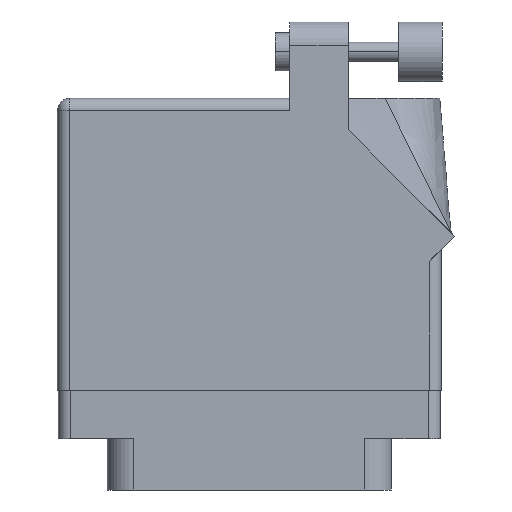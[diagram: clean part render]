
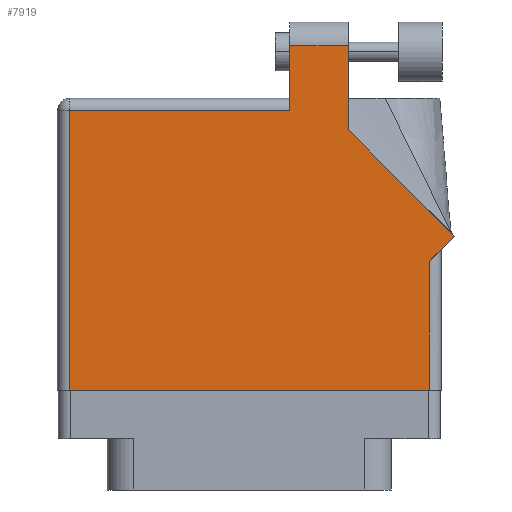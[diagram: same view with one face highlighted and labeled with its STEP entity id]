
A CAD part, front view. The second image highlights one B-rep face of the part: STEP entity #7919.
In plain terms, the highlighted face is planar.
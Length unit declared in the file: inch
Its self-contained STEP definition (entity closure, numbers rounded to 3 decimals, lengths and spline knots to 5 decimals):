
#289 = LINE ( 'NONE', #7121, #29170 ) ;
#647 = CARTESIAN_POINT ( 'NONE',  ( 0.943, 0.575, 0.455 ) ) ;
#1535 = CARTESIAN_POINT ( 'NONE',  ( -1.005, -0.1, 0.455 ) ) ;
#1773 = VECTOR ( 'NONE', #12366, 39.37008 ) ;
#2554 = ORIENTED_EDGE ( 'NONE', *, *, #29920, .T. ) ;
#2751 = CARTESIAN_POINT ( 'NONE',  ( 0.943, -0.1, 0.455 ) ) ;
#2792 = ORIENTED_EDGE ( 'NONE', *, *, #33206, .T. ) ;
#2858 = VECTOR ( 'NONE', #15403, 39.37008 ) ;
#3073 = CARTESIAN_POINT ( 'NONE',  ( 1.07571, 0.70771, 0.455 ) ) ;
#3270 = VERTEX_POINT ( 'NONE', #34535 ) ;
#4361 = VECTOR ( 'NONE', #19715, 39.37008 ) ;
#4856 = VECTOR ( 'NONE', #33491, 39.37008 ) ;
#6023 = EDGE_LOOP ( 'NONE', ( #7789, #2792, #2554, #28616, #22264, #18489, #16115, #16274, #26338 ) ) ;
#7121 = CARTESIAN_POINT ( 'NONE',  ( 0.943, 0.637, 0.455 ) ) ;
#7789 = ORIENTED_EDGE ( 'NONE', *, *, #18440, .T. ) ;
#7872 = LINE ( 'NONE', #28008, #4856 ) ;
#7919 = ADVANCED_FACE ( 'NONE', ( #31712 ), #30090, .F. ) ;
#7931 = DIRECTION ( 'NONE',  ( 0., -1., 0. ) ) ;
#8918 = CARTESIAN_POINT ( 'NONE',  ( 0.519, 1.26442, 0.455 ) ) ;
#8967 = CARTESIAN_POINT ( 'NONE',  ( -1.005, 1.368, 0.455 ) ) ;
#9246 = CARTESIAN_POINT ( 'NONE',  ( -0.943, -0.1, 0.455 ) ) ;
#9746 = EDGE_CURVE ( 'NONE', #3270, #18922, #28383, .T. ) ;
#9978 = VERTEX_POINT ( 'NONE', #35092 ) ;
#10935 = LINE ( 'NONE', #31935, #1773 ) ;
#11515 = LINE ( 'NONE', #20930, #25549 ) ;
#12046 = VECTOR ( 'NONE', #7931, 39.37008 ) ;
#12366 = DIRECTION ( 'NONE',  ( -0.707, 0.707, 0. ) ) ;
#12404 = DIRECTION ( 'NONE',  ( 0., -1., 0. ) ) ;
#12478 = VECTOR ( 'NONE', #12404, 39.37008 ) ;
#15309 = DIRECTION ( 'NONE',  ( 0., 1., 0. ) ) ;
#15403 = DIRECTION ( 'NONE',  ( 0.707, 0.707, 0. ) ) ;
#16115 = ORIENTED_EDGE ( 'NONE', *, *, #29809, .T. ) ;
#16274 = ORIENTED_EDGE ( 'NONE', *, *, #17683, .T. ) ;
#17003 = CARTESIAN_POINT ( 'NONE',  ( -0.943, 1.368, 0.455 ) ) ;
#17367 = VERTEX_POINT ( 'NONE', #2751 ) ;
#17683 = EDGE_CURVE ( 'NONE', #26380, #18165, #27273, .T. ) ;
#18165 = VERTEX_POINT ( 'NONE', #3073 ) ;
#18440 = EDGE_CURVE ( 'NONE', #24172, #9978, #11515, .T. ) ;
#18454 = VERTEX_POINT ( 'NONE', #23887 ) ;
#18489 = ORIENTED_EDGE ( 'NONE', *, *, #34846, .T. ) ;
#18614 = DIRECTION ( 'NONE',  ( 0., 0., -1. ) ) ;
#18792 = CARTESIAN_POINT ( 'NONE',  ( 0.212, 1.43, 0.455 ) ) ;
#18922 = VERTEX_POINT ( 'NONE', #17003 ) ;
#19521 = LINE ( 'NONE', #18792, #12046 ) ;
#19715 = DIRECTION ( 'NONE',  ( -1., 0., 0. ) ) ;
#20930 = CARTESIAN_POINT ( 'NONE',  ( 0.519, 1.26442, 0.455 ) ) ;
#22264 = ORIENTED_EDGE ( 'NONE', *, *, #30363, .T. ) ;
#22865 = AXIS2_PLACEMENT_3D ( 'NONE', #29983, #18614, #32895 ) ;
#23103 = VECTOR ( 'NONE', #32422, 39.37008 ) ;
#23887 = CARTESIAN_POINT ( 'NONE',  ( 0.212, 1.705, 0.455 ) ) ;
#23968 = CARTESIAN_POINT ( 'NONE',  ( 1.005, 0.637, 0.455 ) ) ;
#23973 = CARTESIAN_POINT ( 'NONE',  ( -0.943, -0.1, 0.455 ) ) ;
#24172 = VERTEX_POINT ( 'NONE', #8918 ) ;
#24320 = DIRECTION ( 'NONE',  ( 0., 1., 0. ) ) ;
#25549 = VECTOR ( 'NONE', #15309, 39.37008 ) ;
#26338 = ORIENTED_EDGE ( 'NONE', *, *, #32901, .T. ) ;
#26380 = VERTEX_POINT ( 'NONE', #647 ) ;
#27273 = LINE ( 'NONE', #23968, #2858 ) ;
#28008 = CARTESIAN_POINT ( 'NONE',  ( 0.212, 1.705, 0.455 ) ) ;
#28383 = LINE ( 'NONE', #8967, #4361 ) ;
#28616 = ORIENTED_EDGE ( 'NONE', *, *, #9746, .T. ) ;
#29170 = VECTOR ( 'NONE', #24320, 39.37008 ) ;
#29809 = EDGE_CURVE ( 'NONE', #17367, #26380, #289, .T. ) ;
#29920 = EDGE_CURVE ( 'NONE', #18454, #3270, #19521, .T. ) ;
#29983 = CARTESIAN_POINT ( 'NONE',  ( -1.005, 1.43, 0.455 ) ) ;
#30090 = PLANE ( 'NONE',  #22865 ) ;
#30363 = EDGE_CURVE ( 'NONE', #18922, #34243, #36080, .T. ) ;
#31712 = FACE_OUTER_BOUND ( 'NONE', #6023, .T. ) ;
#31935 = CARTESIAN_POINT ( 'NONE',  ( 1.07571, 0.70771, 0.455 ) ) ;
#32272 = LINE ( 'NONE', #1535, #23103 ) ;
#32422 = DIRECTION ( 'NONE',  ( 1., 0., 0. ) ) ;
#32895 = DIRECTION ( 'NONE',  ( -1., 0., 0. ) ) ;
#32901 = EDGE_CURVE ( 'NONE', #18165, #24172, #10935, .T. ) ;
#33206 = EDGE_CURVE ( 'NONE', #9978, #18454, #7872, .T. ) ;
#33491 = DIRECTION ( 'NONE',  ( -1., 0., 0. ) ) ;
#34243 = VERTEX_POINT ( 'NONE', #23973 ) ;
#34535 = CARTESIAN_POINT ( 'NONE',  ( 0.212, 1.368, 0.455 ) ) ;
#34846 = EDGE_CURVE ( 'NONE', #34243, #17367, #32272, .T. ) ;
#35092 = CARTESIAN_POINT ( 'NONE',  ( 0.519, 1.705, 0.455 ) ) ;
#36080 = LINE ( 'NONE', #9246, #12478 ) ;
